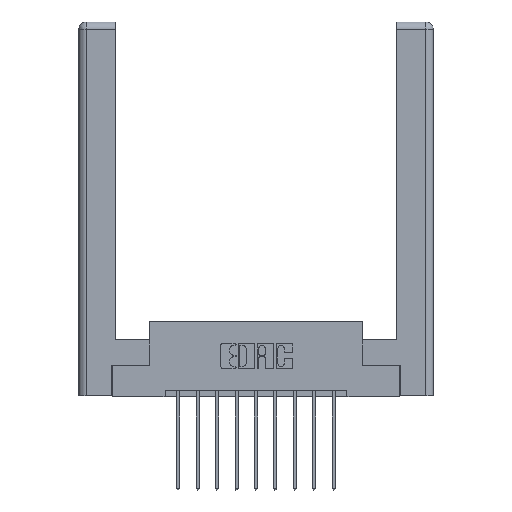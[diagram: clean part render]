
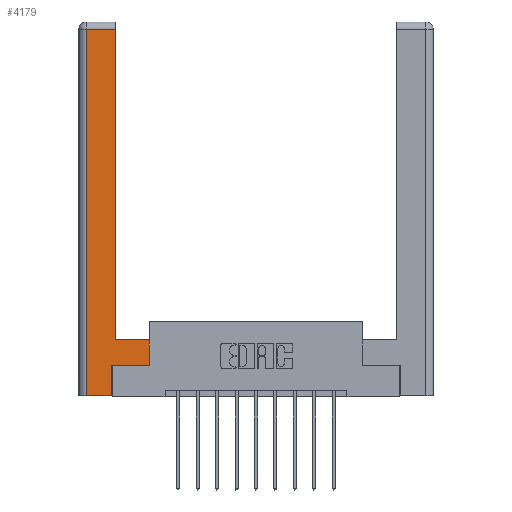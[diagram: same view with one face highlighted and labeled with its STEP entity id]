
A CAD part, top view. The second image highlights one B-rep face of the part: STEP entity #4179.
In plain terms, the highlighted planar face has unit normal (0, 0, 1).
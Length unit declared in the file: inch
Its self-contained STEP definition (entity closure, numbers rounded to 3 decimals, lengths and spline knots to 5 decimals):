
#76 = VERTEX_POINT ( 'NONE', #391 ) ;
#174 = VECTOR ( 'NONE', #5802, 39.37008 ) ;
#391 = CARTESIAN_POINT ( 'NONE',  ( 0.295, 0.45, 0. ) ) ;
#406 = EDGE_CURVE ( 'NONE', #2564, #13292, #6080, .T. ) ;
#605 = VECTOR ( 'NONE', #2345, 39.37008 ) ;
#1018 = VECTOR ( 'NONE', #4008, 39.37008 ) ;
#1054 = ORIENTED_EDGE ( 'NONE', *, *, #9607, .T. ) ;
#1101 = ORIENTED_EDGE ( 'NONE', *, *, #406, .T. ) ;
#1256 = CARTESIAN_POINT ( 'NONE',  ( 0.295, 2.94, 0. ) ) ;
#2040 = VERTEX_POINT ( 'NONE', #4304 ) ;
#2126 = CARTESIAN_POINT ( 'NONE',  ( 0.295, 0.45, 0. ) ) ;
#2345 = DIRECTION ( 'NONE',  ( 0., -1., 0. ) ) ;
#2564 = VERTEX_POINT ( 'NONE', #4955 ) ;
#2600 = VECTOR ( 'NONE', #5504, 39.37008 ) ;
#3437 = DIRECTION ( 'NONE',  ( 0., 1., 0. ) ) ;
#3515 = DIRECTION ( 'NONE',  ( 0., 1., 0. ) ) ;
#3819 = VECTOR ( 'NONE', #8490, 39.37008 ) ;
#3922 = DIRECTION ( 'NONE',  ( -1., 0., 0. ) ) ;
#4008 = DIRECTION ( 'NONE',  ( 1., 0., 0. ) ) ;
#4092 = CARTESIAN_POINT ( 'NONE',  ( 0.565, 0.245, 0. ) ) ;
#4112 = LINE ( 'NONE', #12535, #605 ) ;
#4179 = ADVANCED_FACE ( 'NONE', ( #7844 ), #7415, .F. ) ;
#4304 = CARTESIAN_POINT ( 'NONE',  ( 0.265, 0.245, 0. ) ) ;
#4674 = LINE ( 'NONE', #10995, #5687 ) ;
#4756 = CARTESIAN_POINT ( 'NONE',  ( 0.0615, 2.94, 0. ) ) ;
#4808 = LINE ( 'NONE', #2126, #3819 ) ;
#4955 = CARTESIAN_POINT ( 'NONE',  ( 0.0615, 0., 0. ) ) ;
#5143 = CARTESIAN_POINT ( 'NONE',  ( 0.565, 0.245, 0. ) ) ;
#5266 = EDGE_CURVE ( 'NONE', #9065, #76, #4808, .T. ) ;
#5504 = DIRECTION ( 'NONE',  ( 1., 0., 0. ) ) ;
#5687 = VECTOR ( 'NONE', #3515, 39.37008 ) ;
#5802 = DIRECTION ( 'NONE',  ( 0., 1., 0. ) ) ;
#5850 = EDGE_CURVE ( 'NONE', #9199, #9065, #12177, .T. ) ;
#5883 = LINE ( 'NONE', #12072, #174 ) ;
#6080 = LINE ( 'NONE', #9781, #2600 ) ;
#6205 = EDGE_CURVE ( 'NONE', #6657, #2564, #4112, .T. ) ;
#6484 = VECTOR ( 'NONE', #3437, 39.37008 ) ;
#6657 = VERTEX_POINT ( 'NONE', #4756 ) ;
#6701 = EDGE_LOOP ( 'NONE', ( #12703, #1054, #8728, #1101, #10104, #10781, #10490, #9925 ) ) ;
#7415 = PLANE ( 'NONE',  #10044 ) ;
#7844 = FACE_OUTER_BOUND ( 'NONE', #6701, .T. ) ;
#8027 = CARTESIAN_POINT ( 'NONE',  ( 0.265, 0., 0. ) ) ;
#8464 = DIRECTION ( 'NONE',  ( 0., 0., -1. ) ) ;
#8490 = DIRECTION ( 'NONE',  ( -1., 0., 0. ) ) ;
#8509 = CARTESIAN_POINT ( 'NONE',  ( 0., 0., 0. ) ) ;
#8728 = ORIENTED_EDGE ( 'NONE', *, *, #6205, .T. ) ;
#9065 = VERTEX_POINT ( 'NONE', #11539 ) ;
#9099 = EDGE_CURVE ( 'NONE', #76, #9357, #5883, .T. ) ;
#9199 = VERTEX_POINT ( 'NONE', #5143 ) ;
#9231 = EDGE_CURVE ( 'NONE', #2040, #9199, #10897, .T. ) ;
#9357 = VERTEX_POINT ( 'NONE', #1256 ) ;
#9599 = DIRECTION ( 'NONE',  ( -1., 0., 0. ) ) ;
#9607 = EDGE_CURVE ( 'NONE', #9357, #6657, #11540, .T. ) ;
#9709 = VECTOR ( 'NONE', #3922, 39.37008 ) ;
#9781 = CARTESIAN_POINT ( 'NONE',  ( 0.265, 0., 0. ) ) ;
#9925 = ORIENTED_EDGE ( 'NONE', *, *, #5266, .T. ) ;
#10044 = AXIS2_PLACEMENT_3D ( 'NONE', #8509, #8464, #9599 ) ;
#10104 = ORIENTED_EDGE ( 'NONE', *, *, #10406, .T. ) ;
#10406 = EDGE_CURVE ( 'NONE', #13292, #2040, #4674, .T. ) ;
#10490 = ORIENTED_EDGE ( 'NONE', *, *, #5850, .T. ) ;
#10781 = ORIENTED_EDGE ( 'NONE', *, *, #9231, .T. ) ;
#10897 = LINE ( 'NONE', #4092, #1018 ) ;
#10995 = CARTESIAN_POINT ( 'NONE',  ( 0.265, 0.245, 0. ) ) ;
#11539 = CARTESIAN_POINT ( 'NONE',  ( 0.565, 0.45, 0. ) ) ;
#11540 = LINE ( 'NONE', #13658, #9709 ) ;
#12072 = CARTESIAN_POINT ( 'NONE',  ( 0.295, 3., 0. ) ) ;
#12092 = CARTESIAN_POINT ( 'NONE',  ( 0.565, 0.45, 0. ) ) ;
#12177 = LINE ( 'NONE', #12092, #6484 ) ;
#12535 = CARTESIAN_POINT ( 'NONE',  ( 0.0615, 0., 0. ) ) ;
#12703 = ORIENTED_EDGE ( 'NONE', *, *, #9099, .T. ) ;
#13292 = VERTEX_POINT ( 'NONE', #8027 ) ;
#13658 = CARTESIAN_POINT ( 'NONE',  ( 0.0615, 2.94, 0. ) ) ;
